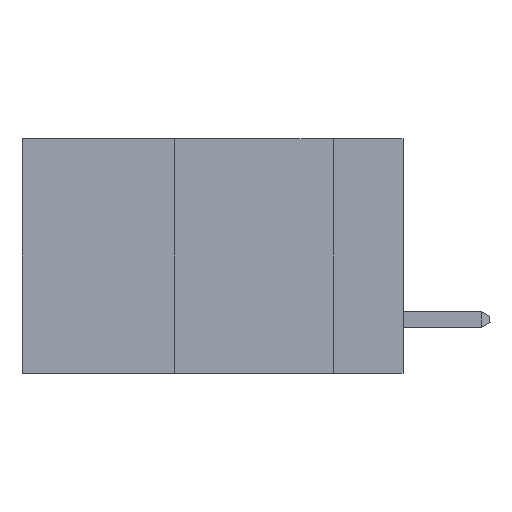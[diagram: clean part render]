
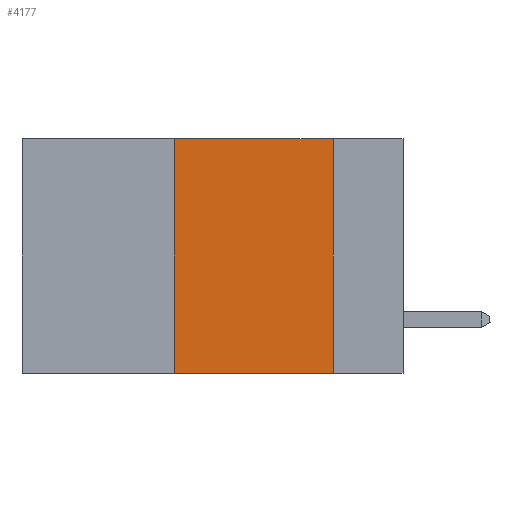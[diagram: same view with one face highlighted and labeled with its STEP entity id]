
A CAD part, left-side view. The second image highlights one B-rep face of the part: STEP entity #4177.
In plain terms, the highlighted planar face has unit normal (-1, 0, 0).
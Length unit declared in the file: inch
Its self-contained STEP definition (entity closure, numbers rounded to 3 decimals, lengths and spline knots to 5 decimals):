
#587 = CARTESIAN_POINT ( 'NONE',  ( 0., 0.36, 0. ) ) ;
#4177 = ADVANCED_FACE ( 'NONE', ( #5813 ), #10856, .F. ) ;
#4458 = CARTESIAN_POINT ( 'NONE',  ( 0., 0.11, 0. ) ) ;
#5240 = DIRECTION ( 'NONE',  ( 1., 0., 0. ) ) ;
#5813 = FACE_OUTER_BOUND ( 'NONE', #17620, .T. ) ;
#7758 = LINE ( 'NONE', #15799, #27528 ) ;
#9258 = AXIS2_PLACEMENT_3D ( 'NONE', #10739, #5240, #36722 ) ;
#10739 = CARTESIAN_POINT ( 'NONE',  ( 0., 0.6, 0. ) ) ;
#10856 = PLANE ( 'NONE',  #9258 ) ;
#11224 = ORIENTED_EDGE ( 'NONE', *, *, #15710, .F. ) ;
#11376 = VERTEX_POINT ( 'NONE', #36674 ) ;
#11844 = ORIENTED_EDGE ( 'NONE', *, *, #21465, .F. ) ;
#12181 = CARTESIAN_POINT ( 'NONE',  ( 0., 0.36, 0. ) ) ;
#15357 = DIRECTION ( 'NONE',  ( 0., 0., 1. ) ) ;
#15710 = EDGE_CURVE ( 'NONE', #11376, #27388, #31754, .T. ) ;
#15799 = CARTESIAN_POINT ( 'NONE',  ( 0., 0.6, -0.37 ) ) ;
#17439 = VERTEX_POINT ( 'NONE', #32430 ) ;
#17620 = EDGE_LOOP ( 'NONE', ( #32501, #11844, #11224, #33308 ) ) ;
#17763 = DIRECTION ( 'NONE',  ( 0., -1., 0. ) ) ;
#18423 = VECTOR ( 'NONE', #17763, 39.37008 ) ;
#18970 = DIRECTION ( 'NONE',  ( 0., -1., 0. ) ) ;
#20430 = VECTOR ( 'NONE', #29143, 39.37008 ) ;
#20580 = CARTESIAN_POINT ( 'NONE',  ( 0., 0.6, 0. ) ) ;
#21465 = EDGE_CURVE ( 'NONE', #27388, #17439, #30658, .T. ) ;
#24149 = CARTESIAN_POINT ( 'NONE',  ( 0., 0.11, -0.37 ) ) ;
#26732 = VECTOR ( 'NONE', #15357, 39.37008 ) ;
#26846 = EDGE_CURVE ( 'NONE', #17439, #28555, #36726, .T. ) ;
#27388 = VERTEX_POINT ( 'NONE', #587 ) ;
#27528 = VECTOR ( 'NONE', #18970, 39.37008 ) ;
#28555 = VERTEX_POINT ( 'NONE', #24149 ) ;
#29143 = DIRECTION ( 'NONE',  ( 0., 0., -1. ) ) ;
#30658 = LINE ( 'NONE', #20580, #18423 ) ;
#31754 = LINE ( 'NONE', #12181, #26732 ) ;
#32430 = CARTESIAN_POINT ( 'NONE',  ( 0., 0.11, 0. ) ) ;
#32501 = ORIENTED_EDGE ( 'NONE', *, *, #26846, .F. ) ;
#33308 = ORIENTED_EDGE ( 'NONE', *, *, #37077, .T. ) ;
#36674 = CARTESIAN_POINT ( 'NONE',  ( 0., 0.36, -0.37 ) ) ;
#36722 = DIRECTION ( 'NONE',  ( 0., 0., -1. ) ) ;
#36726 = LINE ( 'NONE', #4458, #20430 ) ;
#37077 = EDGE_CURVE ( 'NONE', #11376, #28555, #7758, .T. ) ;
